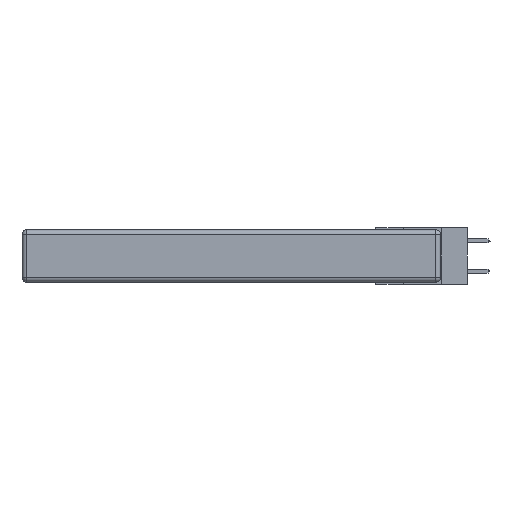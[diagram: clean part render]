
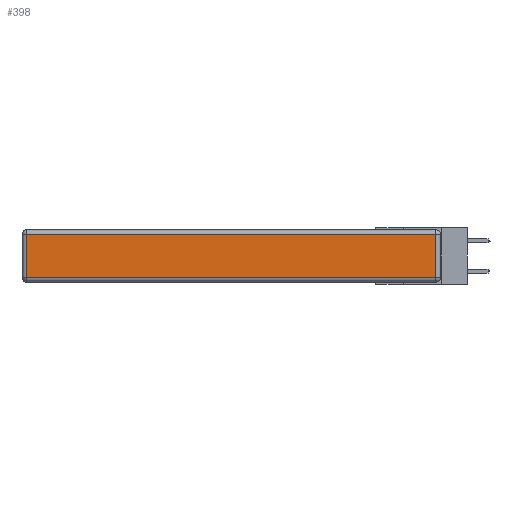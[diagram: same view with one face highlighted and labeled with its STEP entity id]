
A CAD part, left-side view. The second image highlights one B-rep face of the part: STEP entity #398.
In plain terms, the highlighted planar face has unit normal (-1, 0, 0).
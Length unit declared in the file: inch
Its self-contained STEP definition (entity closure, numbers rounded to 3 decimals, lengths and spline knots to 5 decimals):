
#11 = DIRECTION ( 'NONE',  ( 0., 0., 1. ) ) ;
#398 = ADVANCED_FACE ( 'NONE', ( #1298 ), #10520, .T. ) ;
#470 = DIRECTION ( 'NONE',  ( 0., 0., -1. ) ) ;
#553 = CARTESIAN_POINT ( 'NONE',  ( 0., 0.03, -0.313 ) ) ;
#621 = LINE ( 'NONE', #10821, #13598 ) ;
#1298 = FACE_OUTER_BOUND ( 'NONE', #15257, .T. ) ;
#1429 = ORIENTED_EDGE ( 'NONE', *, *, #6811, .T. ) ;
#1459 = EDGE_CURVE ( 'NONE', #8330, #5743, #9600, .T. ) ;
#2166 = ORIENTED_EDGE ( 'NONE', *, *, #16536, .T. ) ;
#3059 = CARTESIAN_POINT ( 'NONE',  ( 0., 0.03, -0.03 ) ) ;
#4473 = DIRECTION ( 'NONE',  ( 0., 0., 1. ) ) ;
#5028 = VERTEX_POINT ( 'NONE', #7604 ) ;
#5451 = AXIS2_PLACEMENT_3D ( 'NONE', #15742, #15683, #11 ) ;
#5743 = VERTEX_POINT ( 'NONE', #3059 ) ;
#5792 = CARTESIAN_POINT ( 'NONE',  ( 0., 0., -0.313 ) ) ;
#6239 = ORIENTED_EDGE ( 'NONE', *, *, #1459, .T. ) ;
#6551 = CARTESIAN_POINT ( 'NONE',  ( 0., 2.75, -0.03 ) ) ;
#6811 = EDGE_CURVE ( 'NONE', #5028, #8330, #7880, .T. ) ;
#7480 = EDGE_CURVE ( 'NONE', #5743, #9309, #13509, .T. ) ;
#7604 = CARTESIAN_POINT ( 'NONE',  ( 0., 2.72, -0.313 ) ) ;
#7620 = ORIENTED_EDGE ( 'NONE', *, *, #7480, .T. ) ;
#7880 = LINE ( 'NONE', #5792, #15729 ) ;
#8330 = VERTEX_POINT ( 'NONE', #553 ) ;
#9309 = VERTEX_POINT ( 'NONE', #16386 ) ;
#9600 = LINE ( 'NONE', #16198, #10818 ) ;
#10520 = PLANE ( 'NONE',  #5451 ) ;
#10818 = VECTOR ( 'NONE', #4473, 39.37008 ) ;
#10821 = CARTESIAN_POINT ( 'NONE',  ( 0., 2.72, -0.343 ) ) ;
#13351 = DIRECTION ( 'NONE',  ( 0., -1., 0. ) ) ;
#13509 = LINE ( 'NONE', #6551, #16507 ) ;
#13598 = VECTOR ( 'NONE', #470, 39.37008 ) ;
#14548 = DIRECTION ( 'NONE',  ( 0., 1., 0. ) ) ;
#15257 = EDGE_LOOP ( 'NONE', ( #1429, #6239, #7620, #2166 ) ) ;
#15683 = DIRECTION ( 'NONE',  ( -1., 0., 0. ) ) ;
#15729 = VECTOR ( 'NONE', #13351, 39.37008 ) ;
#15742 = CARTESIAN_POINT ( 'NONE',  ( 0., 0., -0.343 ) ) ;
#16198 = CARTESIAN_POINT ( 'NONE',  ( 0., 0.03, -0.343 ) ) ;
#16386 = CARTESIAN_POINT ( 'NONE',  ( 0., 2.72, -0.03 ) ) ;
#16507 = VECTOR ( 'NONE', #14548, 39.37008 ) ;
#16536 = EDGE_CURVE ( 'NONE', #9309, #5028, #621, .T. ) ;
